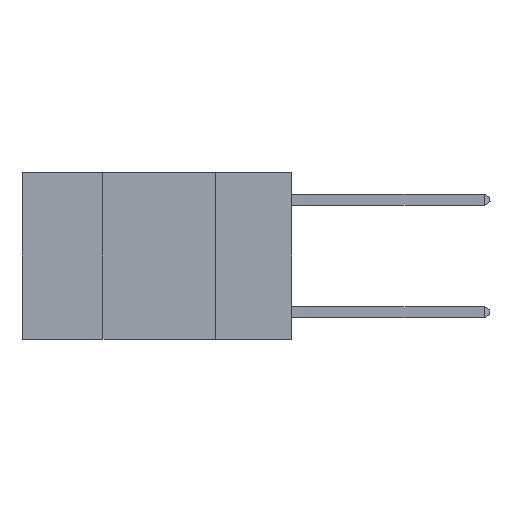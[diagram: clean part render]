
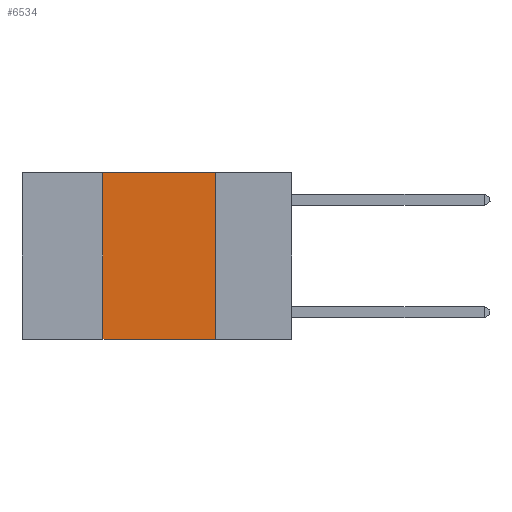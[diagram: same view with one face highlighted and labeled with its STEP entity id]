
A CAD part, left-side view. The second image highlights one B-rep face of the part: STEP entity #6534.
In plain terms, the highlighted planar face has unit normal (-1, 0, 0).
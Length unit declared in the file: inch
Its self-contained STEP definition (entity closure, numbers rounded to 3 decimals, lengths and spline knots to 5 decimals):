
#248 = EDGE_CURVE ( 'NONE', #9327, #1313, #10462, .T. ) ;
#411 = DIRECTION ( 'NONE',  ( 0., -1., 0. ) ) ;
#514 = ORIENTED_EDGE ( 'NONE', *, *, #795, .F. ) ;
#607 = VECTOR ( 'NONE', #10338, 39.37008 ) ;
#640 = ORIENTED_EDGE ( 'NONE', *, *, #248, .F. ) ;
#795 = EDGE_CURVE ( 'NONE', #9368, #7826, #3031, .T. ) ;
#1193 = CARTESIAN_POINT ( 'NONE',  ( 0., 0.17, 0. ) ) ;
#1306 = AXIS2_PLACEMENT_3D ( 'NONE', #2834, #8456, #3636 ) ;
#1313 = VERTEX_POINT ( 'NONE', #2101 ) ;
#1391 = VECTOR ( 'NONE', #9975, 39.37008 ) ;
#2101 = CARTESIAN_POINT ( 'NONE',  ( 0., 0.42, 0. ) ) ;
#2834 = CARTESIAN_POINT ( 'NONE',  ( 0., 0.6, 0. ) ) ;
#3031 = LINE ( 'NONE', #3908, #607 ) ;
#3636 = DIRECTION ( 'NONE',  ( 0., 0., -1. ) ) ;
#3908 = CARTESIAN_POINT ( 'NONE',  ( 0., 0.17, 0. ) ) ;
#4053 = VECTOR ( 'NONE', #411, 39.37008 ) ;
#4422 = EDGE_LOOP ( 'NONE', ( #514, #7951, #640, #7298 ) ) ;
#4447 = CARTESIAN_POINT ( 'NONE',  ( 0., 0.6, -0.37 ) ) ;
#4523 = CARTESIAN_POINT ( 'NONE',  ( 0., 0.6, 0. ) ) ;
#5631 = LINE ( 'NONE', #4447, #4053 ) ;
#5947 = PLANE ( 'NONE',  #1306 ) ;
#6534 = ADVANCED_FACE ( 'NONE', ( #6976 ), #5947, .F. ) ;
#6743 = CARTESIAN_POINT ( 'NONE',  ( 0., 0.17, -0.37 ) ) ;
#6976 = FACE_OUTER_BOUND ( 'NONE', #4422, .T. ) ;
#7298 = ORIENTED_EDGE ( 'NONE', *, *, #9110, .T. ) ;
#7826 = VERTEX_POINT ( 'NONE', #6743 ) ;
#7951 = ORIENTED_EDGE ( 'NONE', *, *, #8535, .F. ) ;
#8456 = DIRECTION ( 'NONE',  ( 1., 0., 0. ) ) ;
#8535 = EDGE_CURVE ( 'NONE', #1313, #9368, #8882, .T. ) ;
#8639 = VECTOR ( 'NONE', #10169, 39.37008 ) ;
#8882 = LINE ( 'NONE', #4523, #8639 ) ;
#9110 = EDGE_CURVE ( 'NONE', #9327, #7826, #5631, .T. ) ;
#9327 = VERTEX_POINT ( 'NONE', #10002 ) ;
#9368 = VERTEX_POINT ( 'NONE', #1193 ) ;
#9618 = CARTESIAN_POINT ( 'NONE',  ( 0., 0.42, 0. ) ) ;
#9975 = DIRECTION ( 'NONE',  ( 0., 0., 1. ) ) ;
#10002 = CARTESIAN_POINT ( 'NONE',  ( 0., 0.42, -0.37 ) ) ;
#10169 = DIRECTION ( 'NONE',  ( 0., -1., 0. ) ) ;
#10338 = DIRECTION ( 'NONE',  ( 0., 0., -1. ) ) ;
#10462 = LINE ( 'NONE', #9618, #1391 ) ;
